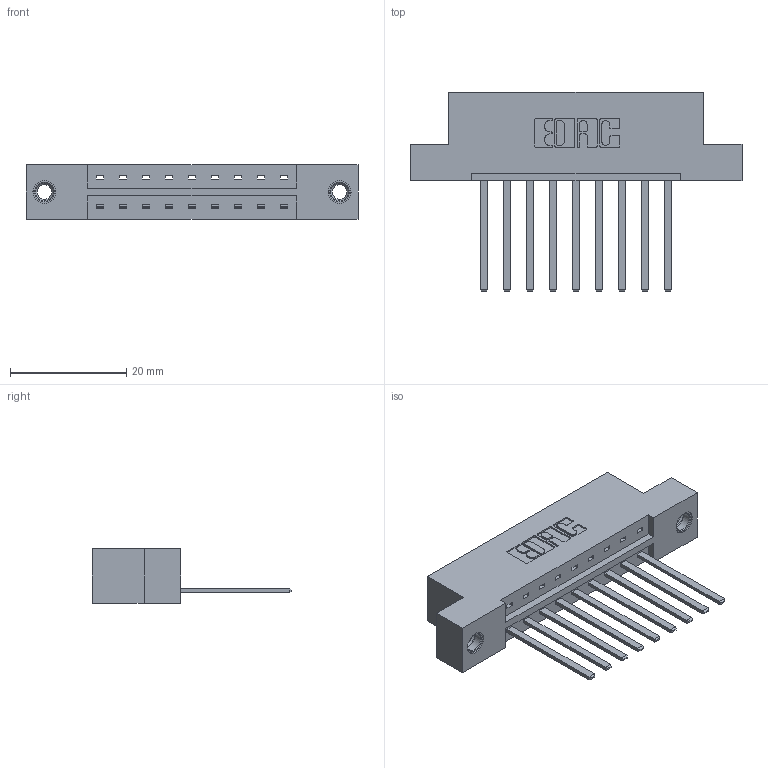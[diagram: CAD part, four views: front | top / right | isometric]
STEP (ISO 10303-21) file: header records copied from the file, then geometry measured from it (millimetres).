
FILE_DESCRIPTION (( 'STEP AP203' ), '1' );
FILE_NAME ('833-009-544-107.STEP', '2020-05-30T17:39:00', ( '' ), ( '' ), 'SwSTEP 2.0', 'SolidWorks 2020', '' );
FILE_SCHEMA (( 'CONFIG_CONTROL_DESIGN' ));
Length unit declared in the file: inch
Products named in the file (4): 345-292-001_345-293-144; 833-009-544-107; 345-250-001_345-250-005-103; 833 Part_Flush - .156 Dia - TI
Assembly tree (12 placements, depth 2):
  833-009-544-107
    833 Part_Flush - .156 Dia - TI
    345-292-001_345-293-144  x9
    345-250-001_345-250-005-103  x2
Bounding box: 57.2 x 34.3 x 9.4 mm (x, y, z)
Volume: 5562.9 mm3; surface area: 6179.4 mm2
Topology: 12 solids, 12 shells, 642 faces, 1869 edges, 1226 vertices
Faces by surface type: plane 444, cylinder 182, cone 12, torus 4
Entity records: 10772 total; most frequent: CARTESIAN_POINT 1844, ORIENTED_EDGE 1782, DIRECTION 1651, EDGE_CURVE 891, VECTOR 747, LINE 747, VERTEX_POINT 588, AXIS2_PLACEMENT_3D 452
